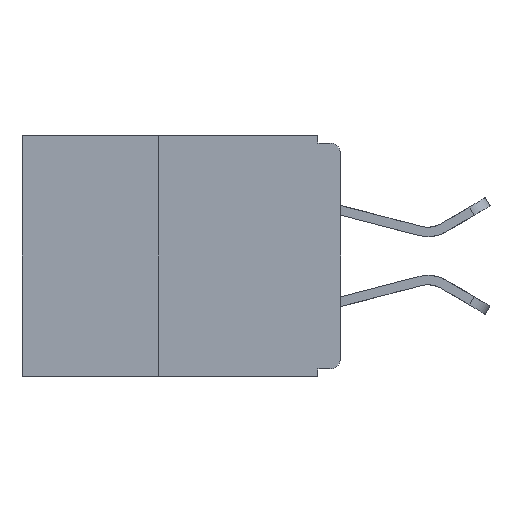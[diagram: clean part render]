
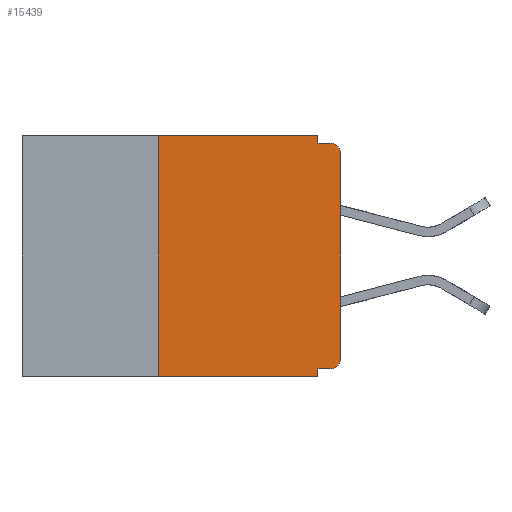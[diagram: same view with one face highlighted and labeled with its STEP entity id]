
A CAD part, left-side view. The second image highlights one B-rep face of the part: STEP entity #15439.
In plain terms, the highlighted planar face has unit normal (-1, 0, 0).
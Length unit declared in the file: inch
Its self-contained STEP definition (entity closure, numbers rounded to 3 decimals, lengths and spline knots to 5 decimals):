
#79 = EDGE_CURVE ( 'NONE', #21840, #13348, #11464, .T. ) ;
#372 = VERTEX_POINT ( 'NONE', #15188 ) ;
#485 = EDGE_CURVE ( 'NONE', #13348, #8441, #11986, .T. ) ;
#760 = DIRECTION ( 'NONE',  ( 0., 0., -1. ) ) ;
#962 = LINE ( 'NONE', #5011, #14824 ) ;
#998 = DIRECTION ( 'NONE',  ( 0., 0., -1. ) ) ;
#1440 = VERTEX_POINT ( 'NONE', #21420 ) ;
#1980 = VECTOR ( 'NONE', #17548, 39.37008 ) ;
#2732 = VECTOR ( 'NONE', #998, 39.37008 ) ;
#3484 = DIRECTION ( 'NONE',  ( 0., 1., 0. ) ) ;
#3658 = VECTOR ( 'NONE', #19400, 39.37008 ) ;
#3862 = CARTESIAN_POINT ( 'NONE',  ( 0., 0.25, -0.33 ) ) ;
#3907 = CARTESIAN_POINT ( 'NONE',  ( 0., 0., -0.01 ) ) ;
#3953 = FACE_OUTER_BOUND ( 'NONE', #9422, .T. ) ;
#4264 = VECTOR ( 'NONE', #18028, 39.37008 ) ;
#4345 = CARTESIAN_POINT ( 'NONE',  ( 0., 0.25, 0. ) ) ;
#4555 = EDGE_CURVE ( 'NONE', #15607, #14249, #17402, .T. ) ;
#4616 = EDGE_CURVE ( 'NONE', #5459, #8441, #7219, .T. ) ;
#4720 = CARTESIAN_POINT ( 'NONE',  ( 0., 0.015, -0.305 ) ) ;
#5011 = CARTESIAN_POINT ( 'NONE',  ( 0., 0.031, 0. ) ) ;
#5459 = VERTEX_POINT ( 'NONE', #3862 ) ;
#5537 = ORIENTED_EDGE ( 'NONE', *, *, #16722, .T. ) ;
#5686 = ORIENTED_EDGE ( 'NONE', *, *, #17927, .T. ) ;
#5831 = ORIENTED_EDGE ( 'NONE', *, *, #12966, .F. ) ;
#6268 = ORIENTED_EDGE ( 'NONE', *, *, #9667, .F. ) ;
#6328 = EDGE_CURVE ( 'NONE', #5459, #15607, #22048, .T. ) ;
#6449 = DIRECTION ( 'NONE',  ( 0., 0., -1. ) ) ;
#6452 = ORIENTED_EDGE ( 'NONE', *, *, #4555, .F. ) ;
#6534 = ORIENTED_EDGE ( 'NONE', *, *, #6328, .F. ) ;
#6633 = ORIENTED_EDGE ( 'NONE', *, *, #4616, .T. ) ;
#6680 = ORIENTED_EDGE ( 'NONE', *, *, #485, .F. ) ;
#6700 = CARTESIAN_POINT ( 'NONE',  ( 0., 0., -0.305 ) ) ;
#6757 = DIRECTION ( 'NONE',  ( 0., 0., -1. ) ) ;
#6783 = EDGE_CURVE ( 'NONE', #21840, #12101, #13067, .T. ) ;
#6863 = CARTESIAN_POINT ( 'NONE',  ( 0., 0.015, -0.32 ) ) ;
#7114 = AXIS2_PLACEMENT_3D ( 'NONE', #14309, #19423, #9246 ) ;
#7219 = LINE ( 'NONE', #17587, #1980 ) ;
#7325 = ORIENTED_EDGE ( 'NONE', *, *, #79, .F. ) ;
#7332 = AXIS2_PLACEMENT_3D ( 'NONE', #21351, #11181, #760 ) ;
#7464 = PLANE ( 'NONE',  #7114 ) ;
#7476 = ORIENTED_EDGE ( 'NONE', *, *, #6783, .T. ) ;
#8441 = VERTEX_POINT ( 'NONE', #20941 ) ;
#8705 = CARTESIAN_POINT ( 'NONE',  ( 0., 0., -0.025 ) ) ;
#9246 = DIRECTION ( 'NONE',  ( 0., 0., -1. ) ) ;
#9422 = EDGE_LOOP ( 'NONE', ( #5537, #5686, #5831, #6268, #6452, #6534, #6633, #6680, #7325, #7476 ) ) ;
#9667 = EDGE_CURVE ( 'NONE', #14249, #372, #962, .T. ) ;
#11181 = DIRECTION ( 'NONE',  ( -1., 0., 0. ) ) ;
#11464 = LINE ( 'NONE', #15131, #16040 ) ;
#11565 = AXIS2_PLACEMENT_3D ( 'NONE', #4720, #16760, #6449 ) ;
#11986 = LINE ( 'NONE', #21511, #2732 ) ;
#12101 = VERTEX_POINT ( 'NONE', #6700 ) ;
#12966 = EDGE_CURVE ( 'NONE', #372, #1440, #12969, .T. ) ;
#12969 = LINE ( 'NONE', #3907, #21440 ) ;
#13067 = CIRCLE ( 'NONE', #11565, 0.015 ) ;
#13348 = VERTEX_POINT ( 'NONE', #15593 ) ;
#13861 = DIRECTION ( 'NONE',  ( 0., 0., 1. ) ) ;
#14003 = LINE ( 'NONE', #14626, #4264 ) ;
#14249 = VERTEX_POINT ( 'NONE', #17841 ) ;
#14309 = CARTESIAN_POINT ( 'NONE',  ( 0., 0.437, 0. ) ) ;
#14626 = CARTESIAN_POINT ( 'NONE',  ( 0., 0., 0. ) ) ;
#14824 = VECTOR ( 'NONE', #6757, 39.37008 ) ;
#15012 = CIRCLE ( 'NONE', #7332, 0.015 ) ;
#15131 = CARTESIAN_POINT ( 'NONE',  ( 0., 0., -0.32 ) ) ;
#15188 = CARTESIAN_POINT ( 'NONE',  ( 0., 0.031, -0.01 ) ) ;
#15439 = ADVANCED_FACE ( 'NONE', ( #3953 ), #7464, .F. ) ;
#15593 = CARTESIAN_POINT ( 'NONE',  ( 0., 0.031, -0.32 ) ) ;
#15607 = VERTEX_POINT ( 'NONE', #4345 ) ;
#16040 = VECTOR ( 'NONE', #3484, 39.37008 ) ;
#16722 = EDGE_CURVE ( 'NONE', #12101, #18781, #14003, .T. ) ;
#16760 = DIRECTION ( 'NONE',  ( -1., 0., 0. ) ) ;
#17054 = CARTESIAN_POINT ( 'NONE',  ( 0., 0.25, -0.33 ) ) ;
#17402 = LINE ( 'NONE', #19754, #3658 ) ;
#17548 = DIRECTION ( 'NONE',  ( 0., -1., 0. ) ) ;
#17587 = CARTESIAN_POINT ( 'NONE',  ( 0., 0.437, -0.33 ) ) ;
#17841 = CARTESIAN_POINT ( 'NONE',  ( 0., 0.031, 0. ) ) ;
#17927 = EDGE_CURVE ( 'NONE', #18781, #1440, #15012, .T. ) ;
#18028 = DIRECTION ( 'NONE',  ( 0., 0., 1. ) ) ;
#18781 = VERTEX_POINT ( 'NONE', #8705 ) ;
#19318 = DIRECTION ( 'NONE',  ( 0., -1., 0. ) ) ;
#19400 = DIRECTION ( 'NONE',  ( 0., -1., 0. ) ) ;
#19423 = DIRECTION ( 'NONE',  ( 1., 0., 0. ) ) ;
#19754 = CARTESIAN_POINT ( 'NONE',  ( 0., 0.437, 0. ) ) ;
#20941 = CARTESIAN_POINT ( 'NONE',  ( 0., 0.031, -0.33 ) ) ;
#21028 = VECTOR ( 'NONE', #13861, 39.37008 ) ;
#21351 = CARTESIAN_POINT ( 'NONE',  ( 0., 0.015, -0.025 ) ) ;
#21420 = CARTESIAN_POINT ( 'NONE',  ( 0., 0.015, -0.01 ) ) ;
#21440 = VECTOR ( 'NONE', #19318, 39.37008 ) ;
#21511 = CARTESIAN_POINT ( 'NONE',  ( 0., 0.031, -0.33 ) ) ;
#21840 = VERTEX_POINT ( 'NONE', #6863 ) ;
#22048 = LINE ( 'NONE', #17054, #21028 ) ;
